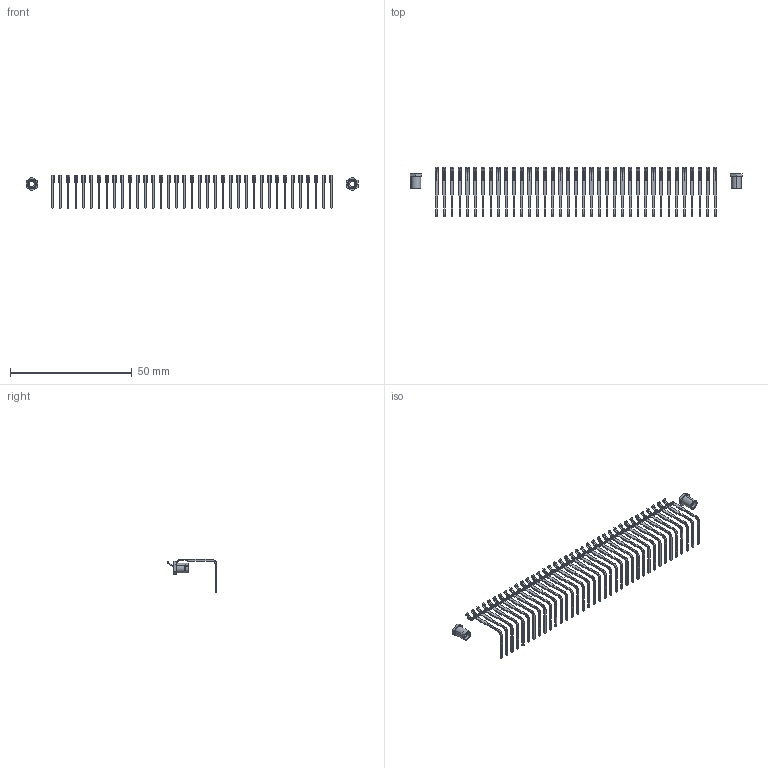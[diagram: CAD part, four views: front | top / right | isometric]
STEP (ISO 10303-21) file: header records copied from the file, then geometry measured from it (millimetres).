
FILE_DESCRIPTION (( 'STEP AP203' ), '1' );
FILE_NAME ('346-037-558-608.STEP', '2018-08-24T03:59:07', ( '' ), ( '' ), 'SwSTEP 2.0', 'SolidWorks 2016', '' );
FILE_SCHEMA (( 'CONFIG_CONTROL_DESIGN' ));
Length unit declared in the file: inch
Products named in the file (4): 346-037-558-608; 346 Part_0.170 Offset - 0.156 Dia-TI; 345-292-001_558 Tail - 2; 345-250-001_345-250-003-102
Assembly tree (40 placements, depth 2):
  346-037-558-608
    346 Part_0.170 Offset - 0.156 Dia-TI
    345-292-001_558 Tail - 2  x37
    345-250-001_345-250-003-102  x2
Bounding box: 136.07 x 20.26 x 13.53 mm (x, y, z)
Volume: 645.8 mm3; surface area: 4004 mm2
Topology: 39 solids, 39 shells, 1822 faces, 5280 edges, 3464 vertices
Faces by surface type: plane 1202, cylinder 604, cone 12, torus 4
Entity records: 25038 total; most frequent: CARTESIAN_POINT 4278, ORIENTED_EDGE 4242, DIRECTION 3805, EDGE_CURVE 2121, LINE 1821, VECTOR 1821, VERTEX_POINT 1408, AXIS2_PLACEMENT_3D 992
